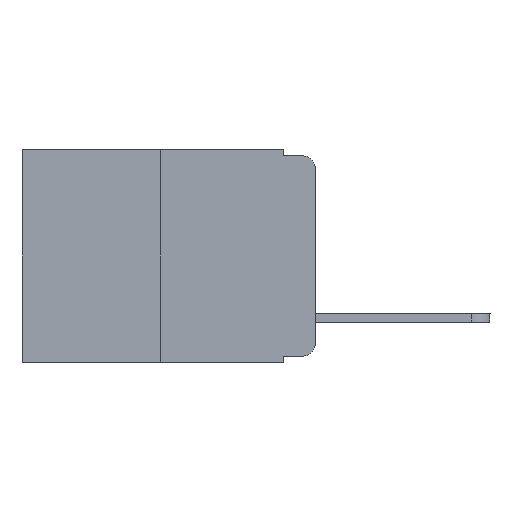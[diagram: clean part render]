
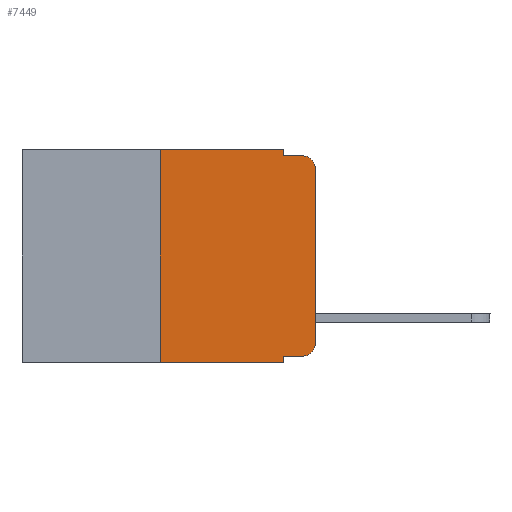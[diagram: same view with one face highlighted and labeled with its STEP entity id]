
A CAD part, left-side view. The second image highlights one B-rep face of the part: STEP entity #7449.
In plain terms, the highlighted planar face has unit normal (-1, 0, 0).
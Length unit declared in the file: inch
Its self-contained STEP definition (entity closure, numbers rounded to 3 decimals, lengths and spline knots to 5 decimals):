
#503 = DIRECTION ( 'NONE',  ( 0., 0., -1. ) ) ;
#1217 = CARTESIAN_POINT ( 'NONE',  ( 0., 0.473, 0. ) ) ;
#1278 = ORIENTED_EDGE ( 'NONE', *, *, #2678, .T. ) ;
#1313 = DIRECTION ( 'NONE',  ( 0., -1., 0. ) ) ;
#1490 = VERTEX_POINT ( 'NONE', #3510 ) ;
#1603 = CARTESIAN_POINT ( 'NONE',  ( 0., 0.02, -0.313 ) ) ;
#1887 = CARTESIAN_POINT ( 'NONE',  ( 0., 0.25, 0. ) ) ;
#2067 = DIRECTION ( 'NONE',  ( 0., 0., 1. ) ) ;
#2158 = EDGE_CURVE ( 'NONE', #11289, #1490, #8580, .T. ) ;
#2557 = LINE ( 'NONE', #1887, #6785 ) ;
#2678 = EDGE_CURVE ( 'NONE', #9927, #11083, #6335, .T. ) ;
#2739 = VERTEX_POINT ( 'NONE', #5318 ) ;
#3001 = EDGE_CURVE ( 'NONE', #10855, #1490, #8207, .T. ) ;
#3028 = EDGE_CURVE ( 'NONE', #2739, #4018, #9365, .T. ) ;
#3089 = ORIENTED_EDGE ( 'NONE', *, *, #3028, .F. ) ;
#3100 = VECTOR ( 'NONE', #11703, 39.37008 ) ;
#3510 = CARTESIAN_POINT ( 'NONE',  ( 0., 0.02, -0.01 ) ) ;
#3580 = LINE ( 'NONE', #10042, #3100 ) ;
#3769 = LINE ( 'NONE', #4730, #10313 ) ;
#3914 = CARTESIAN_POINT ( 'NONE',  ( 0., 0.051, -0.333 ) ) ;
#3959 = CARTESIAN_POINT ( 'NONE',  ( 0., 0., 0. ) ) ;
#4018 = VERTEX_POINT ( 'NONE', #11341 ) ;
#4116 = EDGE_CURVE ( 'NONE', #11322, #5150, #3580, .T. ) ;
#4249 = FACE_OUTER_BOUND ( 'NONE', #4423, .T. ) ;
#4423 = EDGE_LOOP ( 'NONE', ( #7301, #11657, #7982, #10380, #3089, #7491, #6966, #10871, #9409, #1278 ) ) ;
#4529 = DIRECTION ( 'NONE',  ( -1., 0., 0. ) ) ;
#4698 = EDGE_CURVE ( 'NONE', #5472, #5150, #3769, .T. ) ;
#4730 = CARTESIAN_POINT ( 'NONE',  ( 0., 0.051, 0. ) ) ;
#4768 = CARTESIAN_POINT ( 'NONE',  ( 0., 0.051, -0.343 ) ) ;
#4999 = AXIS2_PLACEMENT_3D ( 'NONE', #7773, #8601, #8534 ) ;
#5029 = LINE ( 'NONE', #8760, #7454 ) ;
#5150 = VERTEX_POINT ( 'NONE', #4768 ) ;
#5289 = CARTESIAN_POINT ( 'NONE',  ( 0., 0.473, 0. ) ) ;
#5318 = CARTESIAN_POINT ( 'NONE',  ( 0., 0.25, 0. ) ) ;
#5472 = VERTEX_POINT ( 'NONE', #3914 ) ;
#5647 = CARTESIAN_POINT ( 'NONE',  ( 0., 0., -0.313 ) ) ;
#6005 = CARTESIAN_POINT ( 'NONE',  ( 0., 0.051, -0.01 ) ) ;
#6023 = AXIS2_PLACEMENT_3D ( 'NONE', #5289, #11652, #6236 ) ;
#6236 = DIRECTION ( 'NONE',  ( 0., 0., -1. ) ) ;
#6335 = CIRCLE ( 'NONE', #7105, 0.02 ) ;
#6436 = DIRECTION ( 'NONE',  ( 0., 0., 1. ) ) ;
#6785 = VECTOR ( 'NONE', #6436, 39.37008 ) ;
#6798 = DIRECTION ( 'NONE',  ( 0., -1., 0. ) ) ;
#6966 = ORIENTED_EDGE ( 'NONE', *, *, #4116, .T. ) ;
#7105 = AXIS2_PLACEMENT_3D ( 'NONE', #1603, #4529, #9739 ) ;
#7288 = VECTOR ( 'NONE', #6798, 39.37008 ) ;
#7301 = ORIENTED_EDGE ( 'NONE', *, *, #9769, .T. ) ;
#7420 = CARTESIAN_POINT ( 'NONE',  ( 0., 0.051, -0.333 ) ) ;
#7449 = ADVANCED_FACE ( 'NONE', ( #4249 ), #9877, .F. ) ;
#7454 = VECTOR ( 'NONE', #503, 39.37008 ) ;
#7480 = LINE ( 'NONE', #7420, #7911 ) ;
#7491 = ORIENTED_EDGE ( 'NONE', *, *, #9645, .F. ) ;
#7524 = DIRECTION ( 'NONE',  ( 0., 0., -1. ) ) ;
#7583 = DIRECTION ( 'NONE',  ( 0., -1., 0. ) ) ;
#7773 = CARTESIAN_POINT ( 'NONE',  ( 0., 0.02, -0.03 ) ) ;
#7911 = VECTOR ( 'NONE', #7583, 39.37008 ) ;
#7982 = ORIENTED_EDGE ( 'NONE', *, *, #2158, .F. ) ;
#8123 = CARTESIAN_POINT ( 'NONE',  ( 0., 0., -0.03 ) ) ;
#8207 = CIRCLE ( 'NONE', #4999, 0.02 ) ;
#8407 = LINE ( 'NONE', #3959, #10144 ) ;
#8507 = EDGE_CURVE ( 'NONE', #5472, #9927, #7480, .T. ) ;
#8534 = DIRECTION ( 'NONE',  ( 0., 0., -1. ) ) ;
#8580 = LINE ( 'NONE', #11229, #10822 ) ;
#8601 = DIRECTION ( 'NONE',  ( -1., 0., 0. ) ) ;
#8760 = CARTESIAN_POINT ( 'NONE',  ( 0., 0.051, 0. ) ) ;
#9365 = LINE ( 'NONE', #1217, #7288 ) ;
#9409 = ORIENTED_EDGE ( 'NONE', *, *, #8507, .T. ) ;
#9645 = EDGE_CURVE ( 'NONE', #11322, #2739, #2557, .T. ) ;
#9739 = DIRECTION ( 'NONE',  ( 0., 0., -1. ) ) ;
#9769 = EDGE_CURVE ( 'NONE', #11083, #10855, #8407, .T. ) ;
#9877 = PLANE ( 'NONE',  #6023 ) ;
#9884 = CARTESIAN_POINT ( 'NONE',  ( 0., 0.25, -0.343 ) ) ;
#9927 = VERTEX_POINT ( 'NONE', #11356 ) ;
#10042 = CARTESIAN_POINT ( 'NONE',  ( 0., 0.473, -0.343 ) ) ;
#10144 = VECTOR ( 'NONE', #2067, 39.37008 ) ;
#10313 = VECTOR ( 'NONE', #7524, 39.37008 ) ;
#10380 = ORIENTED_EDGE ( 'NONE', *, *, #11582, .F. ) ;
#10822 = VECTOR ( 'NONE', #1313, 39.37008 ) ;
#10855 = VERTEX_POINT ( 'NONE', #8123 ) ;
#10871 = ORIENTED_EDGE ( 'NONE', *, *, #4698, .F. ) ;
#11083 = VERTEX_POINT ( 'NONE', #5647 ) ;
#11229 = CARTESIAN_POINT ( 'NONE',  ( 0., 0.051, -0.01 ) ) ;
#11289 = VERTEX_POINT ( 'NONE', #6005 ) ;
#11322 = VERTEX_POINT ( 'NONE', #9884 ) ;
#11341 = CARTESIAN_POINT ( 'NONE',  ( 0., 0.051, 0. ) ) ;
#11356 = CARTESIAN_POINT ( 'NONE',  ( 0., 0.02, -0.333 ) ) ;
#11582 = EDGE_CURVE ( 'NONE', #4018, #11289, #5029, .T. ) ;
#11652 = DIRECTION ( 'NONE',  ( 1., 0., 0. ) ) ;
#11657 = ORIENTED_EDGE ( 'NONE', *, *, #3001, .T. ) ;
#11703 = DIRECTION ( 'NONE',  ( 0., -1., 0. ) ) ;
